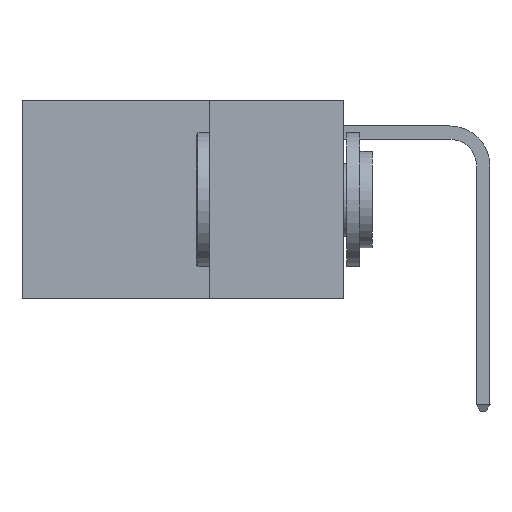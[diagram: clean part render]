
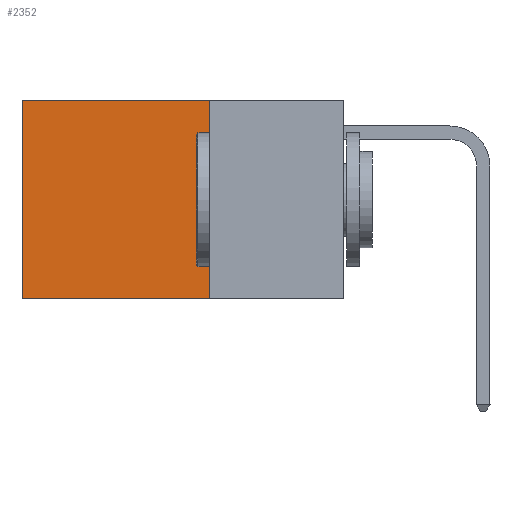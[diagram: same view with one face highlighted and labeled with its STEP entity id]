
A CAD part, left-side view. The second image highlights one B-rep face of the part: STEP entity #2352.
In plain terms, the highlighted planar face has unit normal (-1, 0, 0).
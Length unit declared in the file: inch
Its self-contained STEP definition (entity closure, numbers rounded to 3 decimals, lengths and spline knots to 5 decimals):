
#1017 = CARTESIAN_POINT ( 'NONE',  ( 0.2625, 0.6, -0.37 ) ) ;
#1631 = LINE ( 'NONE', #4183, #4801 ) ;
#2162 = LINE ( 'NONE', #3792, #2448 ) ;
#2352 = ADVANCED_FACE ( 'NONE', ( #4239 ), #2774, .F. ) ;
#2448 = VECTOR ( 'NONE', #5394, 39.37008 ) ;
#2774 = PLANE ( 'NONE',  #7860 ) ;
#3077 = EDGE_CURVE ( 'NONE', #7649, #5675, #9095, .T. ) ;
#3258 = EDGE_CURVE ( 'NONE', #7649, #4231, #8883, .T. ) ;
#3578 = CARTESIAN_POINT ( 'NONE',  ( 0.2625, 0.6, 0. ) ) ;
#3792 = CARTESIAN_POINT ( 'NONE',  ( 0.2625, 0.25, -0.37 ) ) ;
#3972 = CARTESIAN_POINT ( 'NONE',  ( 0.2625, 0.25, 0. ) ) ;
#4040 = CARTESIAN_POINT ( 'NONE',  ( 0.2625, 0.25, 0. ) ) ;
#4097 = EDGE_CURVE ( 'NONE', #4231, #6091, #2162, .T. ) ;
#4183 = CARTESIAN_POINT ( 'NONE',  ( 0.2625, 0.6, 0. ) ) ;
#4231 = VERTEX_POINT ( 'NONE', #8248 ) ;
#4239 = FACE_OUTER_BOUND ( 'NONE', #7390, .T. ) ;
#4579 = VECTOR ( 'NONE', #6767, 39.37008 ) ;
#4801 = VECTOR ( 'NONE', #9039, 39.37008 ) ;
#4836 = ORIENTED_EDGE ( 'NONE', *, *, #4097, .F. ) ;
#5183 = CARTESIAN_POINT ( 'NONE',  ( 0.2625, 0.25, 0. ) ) ;
#5394 = DIRECTION ( 'NONE',  ( 0., 1., 0. ) ) ;
#5675 = VERTEX_POINT ( 'NONE', #3578 ) ;
#6091 = VERTEX_POINT ( 'NONE', #1017 ) ;
#6178 = ORIENTED_EDGE ( 'NONE', *, *, #6509, .T. ) ;
#6328 = DIRECTION ( 'NONE',  ( 0., 0., -1. ) ) ;
#6509 = EDGE_CURVE ( 'NONE', #5675, #6091, #1631, .T. ) ;
#6767 = DIRECTION ( 'NONE',  ( 0., 1., 0. ) ) ;
#7390 = EDGE_LOOP ( 'NONE', ( #6178, #4836, #9486, #10239 ) ) ;
#7462 = CARTESIAN_POINT ( 'NONE',  ( 0.2625, 0.25, 0. ) ) ;
#7649 = VERTEX_POINT ( 'NONE', #4040 ) ;
#7738 = DIRECTION ( 'NONE',  ( 1., 0., 0. ) ) ;
#7860 = AXIS2_PLACEMENT_3D ( 'NONE', #5183, #7738, #8374 ) ;
#8232 = VECTOR ( 'NONE', #6328, 39.37008 ) ;
#8248 = CARTESIAN_POINT ( 'NONE',  ( 0.2625, 0.25, -0.37 ) ) ;
#8374 = DIRECTION ( 'NONE',  ( 0., 0., -1. ) ) ;
#8883 = LINE ( 'NONE', #3972, #8232 ) ;
#9039 = DIRECTION ( 'NONE',  ( 0., 0., -1. ) ) ;
#9095 = LINE ( 'NONE', #7462, #4579 ) ;
#9486 = ORIENTED_EDGE ( 'NONE', *, *, #3258, .F. ) ;
#10239 = ORIENTED_EDGE ( 'NONE', *, *, #3077, .T. ) ;
